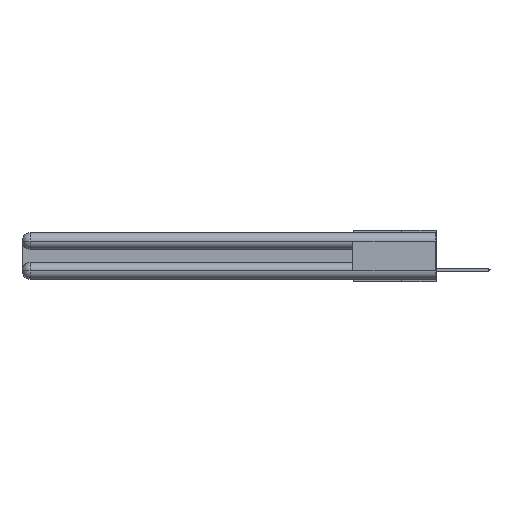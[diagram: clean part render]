
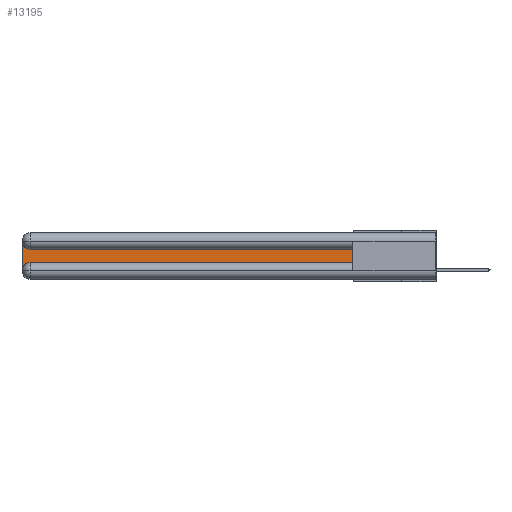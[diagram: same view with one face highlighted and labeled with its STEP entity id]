
A CAD part, left-side view. The second image highlights one B-rep face of the part: STEP entity #13195.
In plain terms, the highlighted planar face has unit normal (-1, 0, 0).
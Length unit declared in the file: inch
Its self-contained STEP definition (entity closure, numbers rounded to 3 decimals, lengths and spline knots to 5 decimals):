
#871 = CIRCLE ( 'NONE', #31116, 0.06 ) ;
#1558 = EDGE_CURVE ( 'NONE', #29166, #24588, #15641, .T. ) ;
#2793 = CARTESIAN_POINT ( 'NONE',  ( 0.075, 2.94, -0.2175 ) ) ;
#3977 = CIRCLE ( 'NONE', #24471, 0.06 ) ;
#4069 = VERTEX_POINT ( 'NONE', #22410 ) ;
#4741 = ORIENTED_EDGE ( 'NONE', *, *, #28339, .T. ) ;
#4799 = DIRECTION ( 'NONE',  ( 1., 0., 0. ) ) ;
#7353 = DIRECTION ( 'NONE',  ( 0., 0., -1. ) ) ;
#7388 = DIRECTION ( 'NONE',  ( 0., -1., 0. ) ) ;
#8138 = ORIENTED_EDGE ( 'NONE', *, *, #1558, .T. ) ;
#9150 = EDGE_CURVE ( 'NONE', #28766, #30377, #3977, .T. ) ;
#9443 = CARTESIAN_POINT ( 'NONE',  ( 0.075, 0.6, -0.2175 ) ) ;
#9444 = CARTESIAN_POINT ( 'NONE',  ( 0.075, 0.6, -0.1225 ) ) ;
#10067 = VECTOR ( 'NONE', #20915, 39.37008 ) ;
#10252 = LINE ( 'NONE', #9443, #18720 ) ;
#10599 = VECTOR ( 'NONE', #7388, 39.37008 ) ;
#10892 = ORIENTED_EDGE ( 'NONE', *, *, #14493, .T. ) ;
#12099 = PLANE ( 'NONE',  #25976 ) ;
#12536 = ORIENTED_EDGE ( 'NONE', *, *, #17286, .T. ) ;
#13195 = ADVANCED_FACE ( 'NONE', ( #13712 ), #12099, .F. ) ;
#13712 = FACE_OUTER_BOUND ( 'NONE', #15092, .T. ) ;
#14027 = CARTESIAN_POINT ( 'NONE',  ( 0.075, 3., -0.0625 ) ) ;
#14204 = DIRECTION ( 'NONE',  ( 0., 1., 0. ) ) ;
#14493 = EDGE_CURVE ( 'NONE', #30344, #28766, #26717, .T. ) ;
#15092 = EDGE_LOOP ( 'NONE', ( #10892, #31295, #4741, #12536, #8138, #22468 ) ) ;
#15428 = CARTESIAN_POINT ( 'NONE',  ( 0.075, 0.6, -0.2175 ) ) ;
#15641 = LINE ( 'NONE', #29654, #10599 ) ;
#16603 = DIRECTION ( 'NONE',  ( 0., 0., -1. ) ) ;
#17286 = EDGE_CURVE ( 'NONE', #4069, #29166, #871, .T. ) ;
#18419 = CARTESIAN_POINT ( 'NONE',  ( 0.075, 3., -0.2175 ) ) ;
#18645 = VECTOR ( 'NONE', #14204, 39.37008 ) ;
#18720 = VECTOR ( 'NONE', #22051, 39.37008 ) ;
#20915 = DIRECTION ( 'NONE',  ( 0., 0., -1. ) ) ;
#21574 = CARTESIAN_POINT ( 'NONE',  ( 0.075, 2.94, -0.1225 ) ) ;
#22051 = DIRECTION ( 'NONE',  ( 0., 0., 1. ) ) ;
#22410 = CARTESIAN_POINT ( 'NONE',  ( 0.075, 3., -0.2775 ) ) ;
#22468 = ORIENTED_EDGE ( 'NONE', *, *, #24468, .T. ) ;
#23910 = LINE ( 'NONE', #18419, #10067 ) ;
#24468 = EDGE_CURVE ( 'NONE', #24588, #30344, #10252, .T. ) ;
#24471 = AXIS2_PLACEMENT_3D ( 'NONE', #26253, #31400, #16603 ) ;
#24513 = DIRECTION ( 'NONE',  ( 0., 0., -1. ) ) ;
#24588 = VERTEX_POINT ( 'NONE', #15428 ) ;
#25976 = AXIS2_PLACEMENT_3D ( 'NONE', #29721, #31813, #7353 ) ;
#26253 = CARTESIAN_POINT ( 'NONE',  ( 0.075, 2.94, -0.0625 ) ) ;
#26283 = CARTESIAN_POINT ( 'NONE',  ( 0.075, 0.6, -0.1225 ) ) ;
#26717 = LINE ( 'NONE', #9444, #18645 ) ;
#28339 = EDGE_CURVE ( 'NONE', #30377, #4069, #23910, .T. ) ;
#28766 = VERTEX_POINT ( 'NONE', #21574 ) ;
#29166 = VERTEX_POINT ( 'NONE', #2793 ) ;
#29305 = CARTESIAN_POINT ( 'NONE',  ( 0.075, 2.94, -0.2775 ) ) ;
#29654 = CARTESIAN_POINT ( 'NONE',  ( 0.075, 0.6, -0.2175 ) ) ;
#29721 = CARTESIAN_POINT ( 'NONE',  ( 0.075, 3., -0.1225 ) ) ;
#30344 = VERTEX_POINT ( 'NONE', #26283 ) ;
#30377 = VERTEX_POINT ( 'NONE', #14027 ) ;
#31116 = AXIS2_PLACEMENT_3D ( 'NONE', #29305, #4799, #24513 ) ;
#31295 = ORIENTED_EDGE ( 'NONE', *, *, #9150, .T. ) ;
#31400 = DIRECTION ( 'NONE',  ( 1., 0., 0. ) ) ;
#31813 = DIRECTION ( 'NONE',  ( 1., 0., 0. ) ) ;
